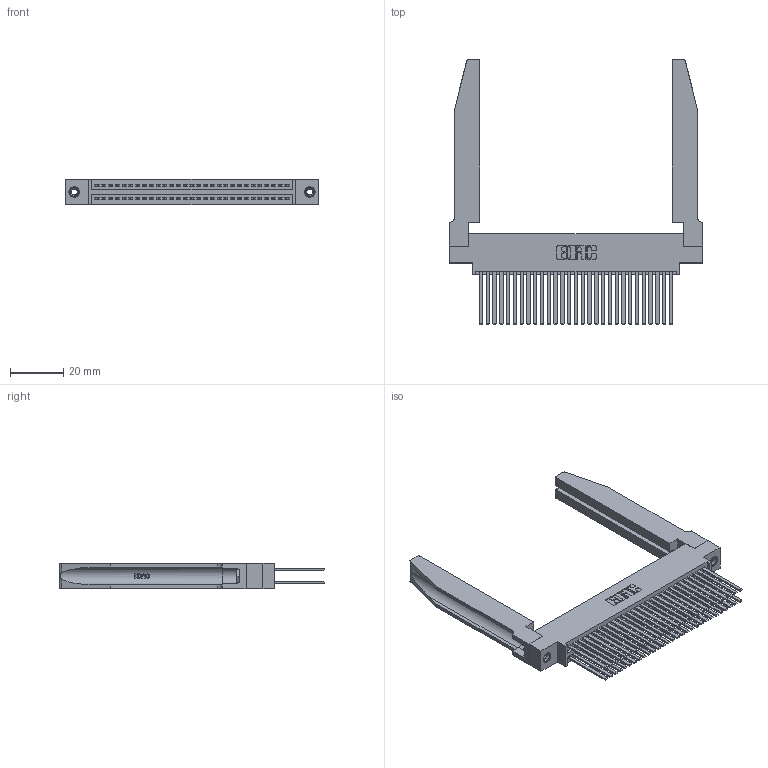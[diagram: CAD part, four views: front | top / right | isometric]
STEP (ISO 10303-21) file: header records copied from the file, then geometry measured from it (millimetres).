
FILE_DESCRIPTION (( 'STEP AP203' ), '1' );
FILE_NAME ('345-058-544-878.STEP', '2019-10-30T05:49:13', ( '' ), ( '' ), 'SwSTEP 2.0', 'SolidWorks 2016', '' );
FILE_SCHEMA (( 'CONFIG_CONTROL_DESIGN' ));
Length unit declared in the file: inch
Products named in the file (5): 345 Part_0.170 Offset - 0.156 Dia-TH; 345-292-001_345-293-144; 345-250-001_345-250-001-102; 345-058-544-878; 345-220-078_345-220-078
Assembly tree (63 placements, depth 2):
  345-058-544-878
    345 Part_0.170 Offset - 0.156 Dia-TH
    345-292-001_345-293-144  x58
    345-250-001_345-250-001-102  x2
    345-220-078_345-220-078  x2
Bounding box: 94.89 x 99.24 x 9.4 mm (x, y, z)
Volume: 17567.6 mm3; surface area: 23594.9 mm2
Topology: 63 solids, 63 shells, 2916 faces, 8559 edges, 5618 vertices
Faces by surface type: plane 1908, cylinder 956, bspline 36, cone 12, torus 4
Entity records: 29192 total; most frequent: CARTESIAN_POINT 5823, ORIENTED_EDGE 4654, DIRECTION 4141, EDGE_CURVE 2327, VECTOR 1989, LINE 1989, VERTEX_POINT 1544, AXIS2_PLACEMENT_3D 1076
